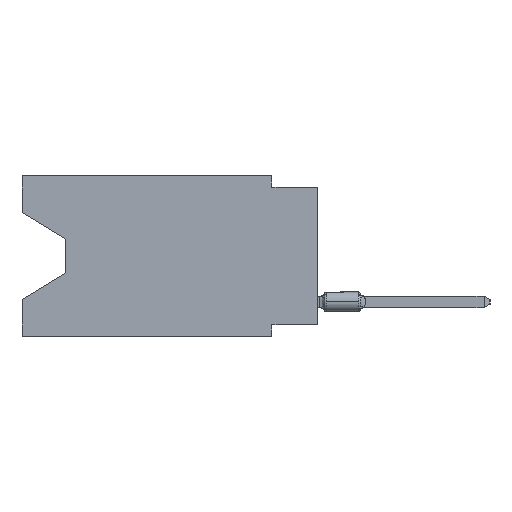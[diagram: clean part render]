
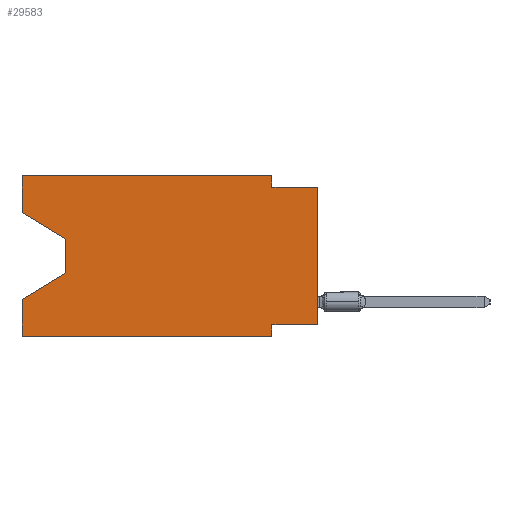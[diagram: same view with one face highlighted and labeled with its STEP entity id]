
A CAD part, left-side view. The second image highlights one B-rep face of the part: STEP entity #29583.
In plain terms, the highlighted planar face has unit normal (-1, 0, 0).
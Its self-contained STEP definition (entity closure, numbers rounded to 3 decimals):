
#893 = FACE_OUTER_BOUND ( 'NONE', #51514, .T. ) ;
#2147 = VECTOR ( 'NONE', #66228, 1000. ) ;
#2327 = LINE ( 'NONE', #51640, #39938 ) ;
#2469 = ORIENTED_EDGE ( 'NONE', *, *, #54004, .F. ) ;
#3901 = ORIENTED_EDGE ( 'NONE', *, *, #37662, .T. ) ;
#4753 = DIRECTION ( 'NONE',  ( 0., 0.855, -0.519 ) ) ;
#5335 = ORIENTED_EDGE ( 'NONE', *, *, #42447, .T. ) ;
#6017 = CARTESIAN_POINT ( 'NONE',  ( 0., 16.383, 0. ) ) ;
#6290 = AXIS2_PLACEMENT_3D ( 'NONE', #6017, #28671, #28302 ) ;
#6314 = EDGE_CURVE ( 'NONE', #42807, #24129, #66312, .T. ) ;
#6380 = PLANE ( 'NONE',  #6290 ) ;
#6993 = CARTESIAN_POINT ( 'NONE',  ( 0., 16.383, -2.038 ) ) ;
#7784 = LINE ( 'NONE', #45156, #44583 ) ;
#9516 = ORIENTED_EDGE ( 'NONE', *, *, #67467, .T. ) ;
#12080 = EDGE_CURVE ( 'NONE', #24129, #29205, #21644, .T. ) ;
#13084 = EDGE_CURVE ( 'NONE', #44365, #48814, #37667, .T. ) ;
#13302 = DIRECTION ( 'NONE',  ( 0., 0., -1. ) ) ;
#15378 = CARTESIAN_POINT ( 'NONE',  ( 0., 0., 0. ) ) ;
#16433 = LINE ( 'NONE', #21910, #42332 ) ;
#21644 = LINE ( 'NONE', #43931, #2147 ) ;
#21824 = CARTESIAN_POINT ( 'NONE',  ( 0., 16.383, 0. ) ) ;
#21910 = CARTESIAN_POINT ( 'NONE',  ( 0., 16.383, -8.89 ) ) ;
#22012 = VECTOR ( 'NONE', #58863, 1000. ) ;
#23411 = ORIENTED_EDGE ( 'NONE', *, *, #27672, .F. ) ;
#24101 = LINE ( 'NONE', #69064, #63523 ) ;
#24129 = VERTEX_POINT ( 'NONE', #61491 ) ;
#25455 = EDGE_CURVE ( 'NONE', #46132, #42807, #7784, .T. ) ;
#25981 = EDGE_CURVE ( 'NONE', #29205, #48814, #67460, .T. ) ;
#26311 = VERTEX_POINT ( 'NONE', #28274 ) ;
#26349 = CARTESIAN_POINT ( 'NONE',  ( 0., 16.383, -6.852 ) ) ;
#27106 = VECTOR ( 'NONE', #33485, 1000. ) ;
#27672 = EDGE_CURVE ( 'NONE', #42194, #26311, #58012, .T. ) ;
#28274 = CARTESIAN_POINT ( 'NONE',  ( 0., 2.54, -8.89 ) ) ;
#28302 = DIRECTION ( 'NONE',  ( 0., 0., -1. ) ) ;
#28671 = DIRECTION ( 'NONE',  ( 1., 0., 0. ) ) ;
#29205 = VERTEX_POINT ( 'NONE', #34792 ) ;
#29429 = VERTEX_POINT ( 'NONE', #26349 ) ;
#29583 = ADVANCED_FACE ( 'NONE', ( #893 ), #6380, .F. ) ;
#31548 = CARTESIAN_POINT ( 'NONE',  ( 0., 0., -8.255 ) ) ;
#31947 = ORIENTED_EDGE ( 'NONE', *, *, #25455, .F. ) ;
#32533 = CARTESIAN_POINT ( 'NONE',  ( 0., 13.97, -5.385 ) ) ;
#33485 = DIRECTION ( 'NONE',  ( 0., -1., 0. ) ) ;
#33545 = ORIENTED_EDGE ( 'NONE', *, *, #6314, .F. ) ;
#33810 = ORIENTED_EDGE ( 'NONE', *, *, #55288, .F. ) ;
#34340 = VECTOR ( 'NONE', #60814, 1000. ) ;
#34792 = CARTESIAN_POINT ( 'NONE',  ( 0., 2.54, -0.635 ) ) ;
#35373 = CARTESIAN_POINT ( 'NONE',  ( 0., 2.54, -8.89 ) ) ;
#37662 = EDGE_CURVE ( 'NONE', #66862, #29429, #60645, .T. ) ;
#37667 = LINE ( 'NONE', #15378, #22012 ) ;
#37879 = LINE ( 'NONE', #64942, #59922 ) ;
#38264 = CARTESIAN_POINT ( 'NONE',  ( 0., 0., -0.635 ) ) ;
#39938 = VECTOR ( 'NONE', #13302, 1000. ) ;
#40101 = VECTOR ( 'NONE', #57645, 1000. ) ;
#40460 = VERTEX_POINT ( 'NONE', #65346 ) ;
#40838 = VECTOR ( 'NONE', #4753, 1000. ) ;
#42194 = VERTEX_POINT ( 'NONE', #51191 ) ;
#42332 = VECTOR ( 'NONE', #44924, 1000. ) ;
#42447 = EDGE_CURVE ( 'NONE', #40460, #26311, #16433, .T. ) ;
#42807 = VERTEX_POINT ( 'NONE', #21824 ) ;
#43931 = CARTESIAN_POINT ( 'NONE',  ( 0., 2.54, 0. ) ) ;
#44365 = VERTEX_POINT ( 'NONE', #31548 ) ;
#44583 = VECTOR ( 'NONE', #46509, 1000. ) ;
#44924 = DIRECTION ( 'NONE',  ( 0., -1., 0. ) ) ;
#45156 = CARTESIAN_POINT ( 'NONE',  ( 0., 16.383, 0. ) ) ;
#46002 = VERTEX_POINT ( 'NONE', #51906 ) ;
#46132 = VERTEX_POINT ( 'NONE', #6993 ) ;
#46509 = DIRECTION ( 'NONE',  ( 0., 0., 1. ) ) ;
#46876 = EDGE_CURVE ( 'NONE', #46002, #66862, #2327, .T. ) ;
#48814 = VERTEX_POINT ( 'NONE', #38264 ) ;
#50116 = CARTESIAN_POINT ( 'NONE',  ( 0., 16.383, -2.038 ) ) ;
#51191 = CARTESIAN_POINT ( 'NONE',  ( 0., 2.54, -8.255 ) ) ;
#51514 = EDGE_LOOP ( 'NONE', ( #9516, #57467, #3901, #2469, #5335, #23411, #33810, #57128, #58001, #68786, #33545, #31947 ) ) ;
#51640 = CARTESIAN_POINT ( 'NONE',  ( 0., 13.97, -3.505 ) ) ;
#51906 = CARTESIAN_POINT ( 'NONE',  ( 0., 13.97, -3.505 ) ) ;
#54004 = EDGE_CURVE ( 'NONE', #40460, #29429, #37879, .T. ) ;
#54673 = DIRECTION ( 'NONE',  ( 0., 0., 1. ) ) ;
#55288 = EDGE_CURVE ( 'NONE', #44365, #42194, #24101, .T. ) ;
#57128 = ORIENTED_EDGE ( 'NONE', *, *, #13084, .T. ) ;
#57467 = ORIENTED_EDGE ( 'NONE', *, *, #46876, .T. ) ;
#57645 = DIRECTION ( 'NONE',  ( 0., 0., -1. ) ) ;
#58001 = ORIENTED_EDGE ( 'NONE', *, *, #25981, .F. ) ;
#58012 = LINE ( 'NONE', #35373, #40101 ) ;
#58434 = DIRECTION ( 'NONE',  ( 0., 1., 0. ) ) ;
#58863 = DIRECTION ( 'NONE',  ( 0., 0., 1. ) ) ;
#59922 = VECTOR ( 'NONE', #54673, 1000. ) ;
#60645 = LINE ( 'NONE', #32533, #40838 ) ;
#60814 = DIRECTION ( 'NONE',  ( 0., -1., 0. ) ) ;
#61090 = DIRECTION ( 'NONE',  ( 0., -0.855, -0.519 ) ) ;
#61185 = VECTOR ( 'NONE', #61090, 1000. ) ;
#61491 = CARTESIAN_POINT ( 'NONE',  ( 0., 2.54, 0. ) ) ;
#63523 = VECTOR ( 'NONE', #58434, 1000. ) ;
#64942 = CARTESIAN_POINT ( 'NONE',  ( 0., 16.383, 0. ) ) ;
#65346 = CARTESIAN_POINT ( 'NONE',  ( 0., 16.383, -8.89 ) ) ;
#66228 = DIRECTION ( 'NONE',  ( 0., 0., -1. ) ) ;
#66312 = LINE ( 'NONE', #67017, #34340 ) ;
#66578 = LINE ( 'NONE', #50116, #61185 ) ;
#66862 = VERTEX_POINT ( 'NONE', #71397 ) ;
#67017 = CARTESIAN_POINT ( 'NONE',  ( 0., 16.383, 0. ) ) ;
#67460 = LINE ( 'NONE', #67821, #27106 ) ;
#67467 = EDGE_CURVE ( 'NONE', #46132, #46002, #66578, .T. ) ;
#67821 = CARTESIAN_POINT ( 'NONE',  ( 0., 0., -0.635 ) ) ;
#68786 = ORIENTED_EDGE ( 'NONE', *, *, #12080, .F. ) ;
#69064 = CARTESIAN_POINT ( 'NONE',  ( 0., 0., -8.255 ) ) ;
#71397 = CARTESIAN_POINT ( 'NONE',  ( 0., 13.97, -5.385 ) ) ;
